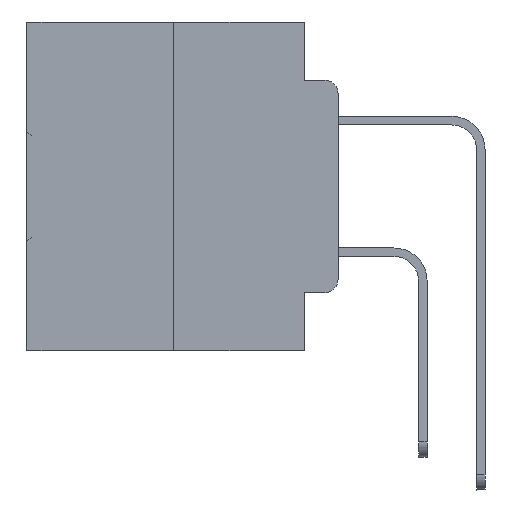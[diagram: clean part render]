
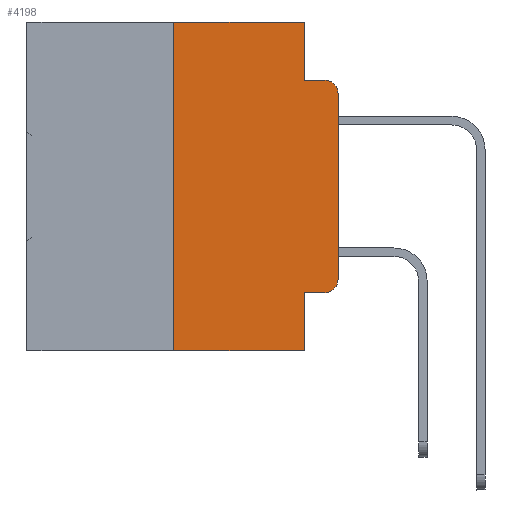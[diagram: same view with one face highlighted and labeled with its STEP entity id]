
A CAD part, left-side view. The second image highlights one B-rep face of the part: STEP entity #4198.
In plain terms, the highlighted planar face has unit normal (-1, 0, 0).
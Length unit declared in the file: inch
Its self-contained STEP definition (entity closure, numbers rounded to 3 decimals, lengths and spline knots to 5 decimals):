
#7 = VERTEX_POINT ( 'NONE', #18275 ) ;
#111 = EDGE_CURVE ( 'NONE', #7, #28500, #25279, .T. ) ;
#966 = DIRECTION ( 'NONE',  ( -1., 0., 0. ) ) ;
#1211 = CARTESIAN_POINT ( 'NONE',  ( 0., 0.051, 0. ) ) ;
#1955 = VERTEX_POINT ( 'NONE', #31729 ) ;
#2116 = VECTOR ( 'NONE', #28916, 39.37008 ) ;
#3573 = ORIENTED_EDGE ( 'NONE', *, *, #23958, .F. ) ;
#3609 = ORIENTED_EDGE ( 'NONE', *, *, #111, .T. ) ;
#4179 = LINE ( 'NONE', #23239, #32680 ) ;
#4198 = ADVANCED_FACE ( 'NONE', ( #9200 ), #24646, .F. ) ;
#4952 = CARTESIAN_POINT ( 'NONE',  ( 0., 0.02, -0.0885 ) ) ;
#5331 = CARTESIAN_POINT ( 'NONE',  ( 0., 0.473, 0. ) ) ;
#5443 = ORIENTED_EDGE ( 'NONE', *, *, #30528, .T. ) ;
#6547 = AXIS2_PLACEMENT_3D ( 'NONE', #17767, #966, #20533 ) ;
#6648 = CARTESIAN_POINT ( 'NONE',  ( 0., 0.02, -0.3915 ) ) ;
#6899 = CIRCLE ( 'NONE', #19422, 0.02 ) ;
#7841 = CARTESIAN_POINT ( 'NONE',  ( 0., 0.051, 0. ) ) ;
#8199 = DIRECTION ( 'NONE',  ( 0., 0., -1. ) ) ;
#8420 = EDGE_CURVE ( 'NONE', #28226, #33457, #13370, .T. ) ;
#8792 = AXIS2_PLACEMENT_3D ( 'NONE', #5331, #24761, #8199 ) ;
#9200 = FACE_OUTER_BOUND ( 'NONE', #14560, .T. ) ;
#9398 = ORIENTED_EDGE ( 'NONE', *, *, #15017, .F. ) ;
#9458 = DIRECTION ( 'NONE',  ( 0., 0., -1. ) ) ;
#9685 = CARTESIAN_POINT ( 'NONE',  ( 0., 0.051, 0. ) ) ;
#10368 = CARTESIAN_POINT ( 'NONE',  ( 0., 0.051, -0.4115 ) ) ;
#10913 = VERTEX_POINT ( 'NONE', #27861 ) ;
#11129 = CARTESIAN_POINT ( 'NONE',  ( 0., 0.051, -0.5 ) ) ;
#11452 = CARTESIAN_POINT ( 'NONE',  ( 0., 0.02, -0.4115 ) ) ;
#12057 = LINE ( 'NONE', #1211, #19435 ) ;
#12812 = CARTESIAN_POINT ( 'NONE',  ( 0., 0.051, -0.4115 ) ) ;
#12855 = ORIENTED_EDGE ( 'NONE', *, *, #28693, .T. ) ;
#13275 = LINE ( 'NONE', #20414, #33362 ) ;
#13370 = LINE ( 'NONE', #10368, #27150 ) ;
#14560 = EDGE_LOOP ( 'NONE', ( #12855, #5443, #18502, #27650, #9398, #16780, #3609, #3573, #18054, #31694 ) ) ;
#14878 = DIRECTION ( 'NONE',  ( 0., -1., 0. ) ) ;
#14996 = CARTESIAN_POINT ( 'NONE',  ( 0., 0.051, -0.0885 ) ) ;
#15017 = EDGE_CURVE ( 'NONE', #1955, #24992, #4179, .T. ) ;
#16355 = VERTEX_POINT ( 'NONE', #31813 ) ;
#16556 = LINE ( 'NONE', #29132, #30249 ) ;
#16780 = ORIENTED_EDGE ( 'NONE', *, *, #22096, .F. ) ;
#17480 = LINE ( 'NONE', #14996, #18336 ) ;
#17523 = CARTESIAN_POINT ( 'NONE',  ( 0., 0., -0.3915 ) ) ;
#17767 = CARTESIAN_POINT ( 'NONE',  ( 0., 0.02, -0.1085 ) ) ;
#18025 = VERTEX_POINT ( 'NONE', #17523 ) ;
#18054 = ORIENTED_EDGE ( 'NONE', *, *, #8420, .T. ) ;
#18275 = CARTESIAN_POINT ( 'NONE',  ( 0., 0.25, -0.5 ) ) ;
#18336 = VECTOR ( 'NONE', #26100, 39.37008 ) ;
#18502 = ORIENTED_EDGE ( 'NONE', *, *, #19562, .F. ) ;
#19270 = CIRCLE ( 'NONE', #6547, 0.02 ) ;
#19422 = AXIS2_PLACEMENT_3D ( 'NONE', #6648, #25995, #9458 ) ;
#19435 = VECTOR ( 'NONE', #20778, 39.37008 ) ;
#19562 = EDGE_CURVE ( 'NONE', #10913, #24991, #17480, .T. ) ;
#20414 = CARTESIAN_POINT ( 'NONE',  ( 0., 0., 0. ) ) ;
#20533 = DIRECTION ( 'NONE',  ( 0., 0., -1. ) ) ;
#20766 = DIRECTION ( 'NONE',  ( 0., -1., 0. ) ) ;
#20778 = DIRECTION ( 'NONE',  ( 0., 0., -1. ) ) ;
#20937 = CARTESIAN_POINT ( 'NONE',  ( 0., 0.473, -0.5 ) ) ;
#21411 = EDGE_CURVE ( 'NONE', #24992, #10913, #23511, .T. ) ;
#22096 = EDGE_CURVE ( 'NONE', #7, #1955, #16556, .T. ) ;
#22714 = VECTOR ( 'NONE', #20766, 39.37008 ) ;
#23205 = DIRECTION ( 'NONE',  ( 0., 0., 1. ) ) ;
#23239 = CARTESIAN_POINT ( 'NONE',  ( 0., 0.473, 0. ) ) ;
#23269 = EDGE_CURVE ( 'NONE', #33457, #18025, #6899, .T. ) ;
#23511 = LINE ( 'NONE', #9685, #2116 ) ;
#23958 = EDGE_CURVE ( 'NONE', #28226, #28500, #12057, .T. ) ;
#24167 = DIRECTION ( 'NONE',  ( 0., -1., 0. ) ) ;
#24646 = PLANE ( 'NONE',  #8792 ) ;
#24761 = DIRECTION ( 'NONE',  ( 1., 0., 0. ) ) ;
#24991 = VERTEX_POINT ( 'NONE', #4952 ) ;
#24992 = VERTEX_POINT ( 'NONE', #7841 ) ;
#25279 = LINE ( 'NONE', #20937, #22714 ) ;
#25995 = DIRECTION ( 'NONE',  ( -1., 0., 0. ) ) ;
#26100 = DIRECTION ( 'NONE',  ( 0., -1., 0. ) ) ;
#27150 = VECTOR ( 'NONE', #24167, 39.37008 ) ;
#27650 = ORIENTED_EDGE ( 'NONE', *, *, #21411, .F. ) ;
#27861 = CARTESIAN_POINT ( 'NONE',  ( 0., 0.051, -0.0885 ) ) ;
#28226 = VERTEX_POINT ( 'NONE', #12812 ) ;
#28500 = VERTEX_POINT ( 'NONE', #11129 ) ;
#28693 = EDGE_CURVE ( 'NONE', #18025, #16355, #13275, .T. ) ;
#28916 = DIRECTION ( 'NONE',  ( 0., 0., -1. ) ) ;
#29132 = CARTESIAN_POINT ( 'NONE',  ( 0., 0.25, 0. ) ) ;
#30249 = VECTOR ( 'NONE', #31846, 39.37008 ) ;
#30528 = EDGE_CURVE ( 'NONE', #16355, #24991, #19270, .T. ) ;
#31694 = ORIENTED_EDGE ( 'NONE', *, *, #23269, .T. ) ;
#31729 = CARTESIAN_POINT ( 'NONE',  ( 0., 0.25, 0. ) ) ;
#31813 = CARTESIAN_POINT ( 'NONE',  ( 0., 0., -0.1085 ) ) ;
#31846 = DIRECTION ( 'NONE',  ( 0., 0., 1. ) ) ;
#32680 = VECTOR ( 'NONE', #14878, 39.37008 ) ;
#33362 = VECTOR ( 'NONE', #23205, 39.37008 ) ;
#33457 = VERTEX_POINT ( 'NONE', #11452 ) ;
